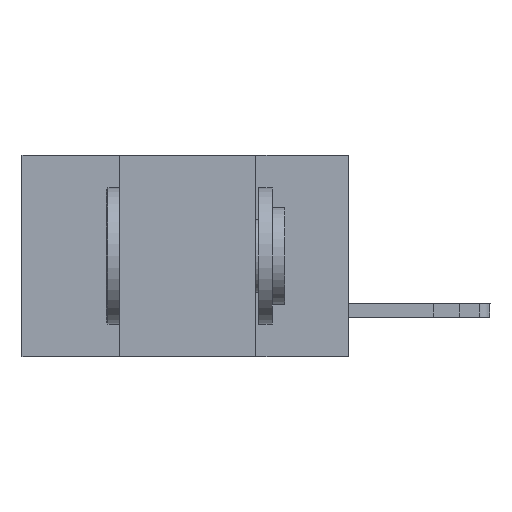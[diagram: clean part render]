
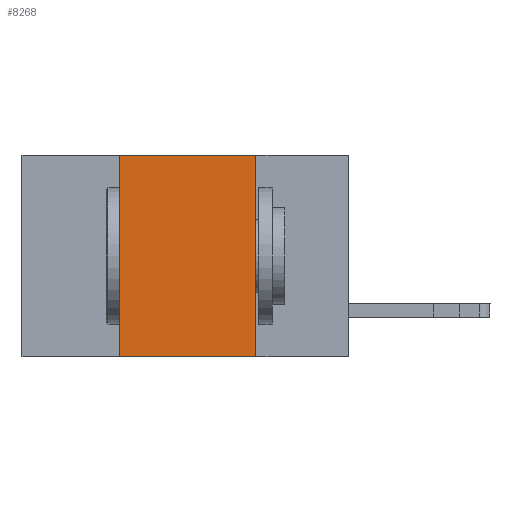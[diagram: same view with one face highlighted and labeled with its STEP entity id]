
A CAD part, left-side view. The second image highlights one B-rep face of the part: STEP entity #8268.
In plain terms, the highlighted planar face has unit normal (-1, 0, 0).
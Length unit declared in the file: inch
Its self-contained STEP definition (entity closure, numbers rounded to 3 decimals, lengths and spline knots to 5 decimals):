
#383 = CARTESIAN_POINT ( 'NONE',  ( 0., 0.6, 0. ) ) ;
#1137 = FACE_OUTER_BOUND ( 'NONE', #19464, .T. ) ;
#1637 = LINE ( 'NONE', #4752, #9733 ) ;
#2147 = ORIENTED_EDGE ( 'NONE', *, *, #17887, .F. ) ;
#4333 = CARTESIAN_POINT ( 'NONE',  ( 0., 0.42, -0.37 ) ) ;
#4752 = CARTESIAN_POINT ( 'NONE',  ( 0., 0.6, -0.37 ) ) ;
#5870 = EDGE_CURVE ( 'NONE', #9039, #9984, #6661, .T. ) ;
#5889 = AXIS2_PLACEMENT_3D ( 'NONE', #19917, #7474, #18477 ) ;
#6661 = LINE ( 'NONE', #18736, #19168 ) ;
#7474 = DIRECTION ( 'NONE',  ( 1., 0., 0. ) ) ;
#8137 = CARTESIAN_POINT ( 'NONE',  ( 0., 0.17, -0.37 ) ) ;
#8268 = ADVANCED_FACE ( 'NONE', ( #1137 ), #16973, .F. ) ;
#8610 = CARTESIAN_POINT ( 'NONE',  ( 0., 0.42, 0. ) ) ;
#9039 = VERTEX_POINT ( 'NONE', #4333 ) ;
#9723 = EDGE_CURVE ( 'NONE', #9039, #19724, #1637, .T. ) ;
#9733 = VECTOR ( 'NONE', #17455, 39.37008 ) ;
#9984 = VERTEX_POINT ( 'NONE', #8610 ) ;
#10453 = LINE ( 'NONE', #14709, #18267 ) ;
#10535 = ORIENTED_EDGE ( 'NONE', *, *, #19895, .F. ) ;
#10966 = ORIENTED_EDGE ( 'NONE', *, *, #5870, .F. ) ;
#11232 = ORIENTED_EDGE ( 'NONE', *, *, #9723, .T. ) ;
#11787 = DIRECTION ( 'NONE',  ( 0., -1., 0. ) ) ;
#14709 = CARTESIAN_POINT ( 'NONE',  ( 0., 0.17, -0.37 ) ) ;
#15392 = VECTOR ( 'NONE', #11787, 39.37008 ) ;
#15864 = LINE ( 'NONE', #383, #15392 ) ;
#16973 = PLANE ( 'NONE',  #5889 ) ;
#17455 = DIRECTION ( 'NONE',  ( 0., -1., 0. ) ) ;
#17700 = VERTEX_POINT ( 'NONE', #20353 ) ;
#17841 = DIRECTION ( 'NONE',  ( 0., 0., 1. ) ) ;
#17887 = EDGE_CURVE ( 'NONE', #17700, #19724, #10453, .T. ) ;
#18267 = VECTOR ( 'NONE', #19248, 39.37008 ) ;
#18477 = DIRECTION ( 'NONE',  ( 0., 0., -1. ) ) ;
#18736 = CARTESIAN_POINT ( 'NONE',  ( 0., 0.42, -0.37 ) ) ;
#19168 = VECTOR ( 'NONE', #17841, 39.37008 ) ;
#19248 = DIRECTION ( 'NONE',  ( 0., 0., -1. ) ) ;
#19464 = EDGE_LOOP ( 'NONE', ( #2147, #10535, #10966, #11232 ) ) ;
#19724 = VERTEX_POINT ( 'NONE', #8137 ) ;
#19895 = EDGE_CURVE ( 'NONE', #9984, #17700, #15864, .T. ) ;
#19917 = CARTESIAN_POINT ( 'NONE',  ( 0., 0.6, 0. ) ) ;
#20353 = CARTESIAN_POINT ( 'NONE',  ( 0., 0.17, 0. ) ) ;
